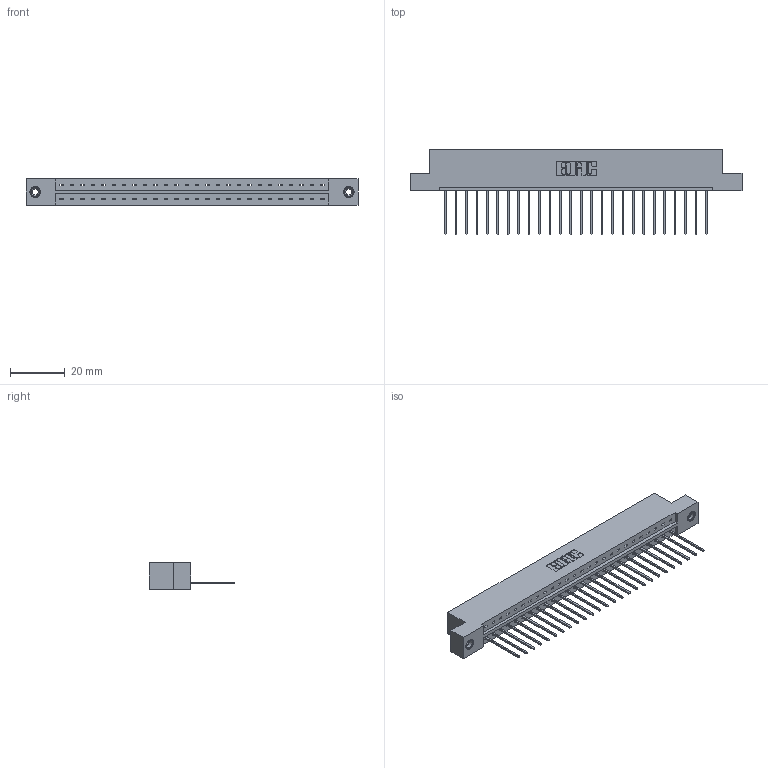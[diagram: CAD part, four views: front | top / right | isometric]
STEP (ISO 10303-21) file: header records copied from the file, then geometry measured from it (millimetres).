
FILE_DESCRIPTION (( 'STEP AP203' ), '1' );
FILE_NAME ('379-026-542-108.STEP', '2020-02-26T15:54:13', ( '' ), ( '' ), 'SwSTEP 2.0', 'SolidWorks 2016', '' );
FILE_SCHEMA (( 'CONFIG_CONTROL_DESIGN' ));
Length unit declared in the file: inch
Products named in the file (4): 379-026-542-108; 345-250-001_345-250-003-102; 345-292-001_345-293-142; 379 Part_Flush - .156 Dia - TI
Assembly tree (29 placements, depth 2):
  379-026-542-108
    379 Part_Flush - .156 Dia - TI
    345-292-001_345-293-142  x26
    345-250-001_345-250-003-102  x2
Bounding box: 121.28 x 31.29 x 9.53 mm (x, y, z)
Volume: 12602.9 mm3; surface area: 13226.5 mm2
Topology: 29 solids, 29 shells, 1682 faces, 5023 edges, 3306 vertices
Faces by surface type: plane 1194, cylinder 472, cone 12, torus 4
Entity records: 19168 total; most frequent: CARTESIAN_POINT 3291, ORIENTED_EDGE 3246, DIRECTION 2841, EDGE_CURVE 1623, LINE 1475, VECTOR 1475, VERTEX_POINT 1076, AXIS2_PLACEMENT_3D 683
